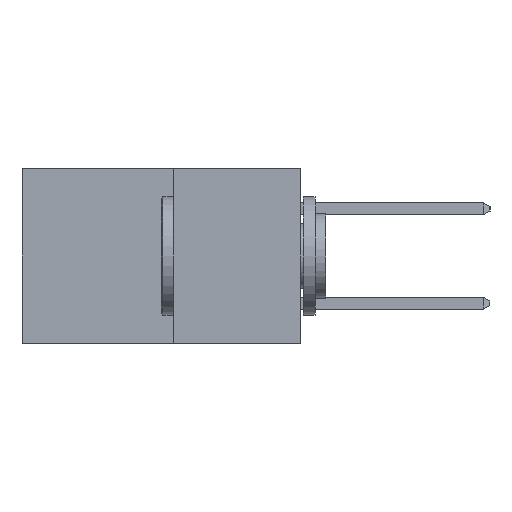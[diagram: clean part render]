
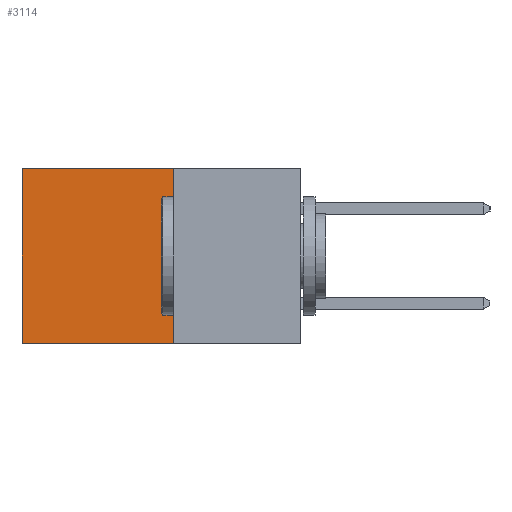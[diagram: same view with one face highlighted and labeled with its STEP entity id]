
A CAD part, left-side view. The second image highlights one B-rep face of the part: STEP entity #3114.
In plain terms, the highlighted planar face has unit normal (-1, 0, 0).
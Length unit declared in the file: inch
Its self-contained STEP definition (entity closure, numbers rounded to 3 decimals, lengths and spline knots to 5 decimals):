
#62 = VECTOR ( 'NONE', #9795, 39.37008 ) ;
#97 = CARTESIAN_POINT ( 'NONE',  ( 0.277, 0.27, -0.37 ) ) ;
#156 = DIRECTION ( 'NONE',  ( 0., 0., -1. ) ) ;
#179 = VECTOR ( 'NONE', #2696, 39.37008 ) ;
#274 = AXIS2_PLACEMENT_3D ( 'NONE', #14590, #12447, #7256 ) ;
#507 = CARTESIAN_POINT ( 'NONE',  ( 0.277, 0.27, -0.37 ) ) ;
#1178 = CARTESIAN_POINT ( 'NONE',  ( 0.277, 0.59, 0. ) ) ;
#2025 = CARTESIAN_POINT ( 'NONE',  ( 0.277, 0.59, -0.37 ) ) ;
#2440 = CARTESIAN_POINT ( 'NONE',  ( 0.277, 0.59, -0.37 ) ) ;
#2696 = DIRECTION ( 'NONE',  ( 0., 1., 0. ) ) ;
#2779 = DIRECTION ( 'NONE',  ( 0., 0., -1. ) ) ;
#2876 = LINE ( 'NONE', #10697, #179 ) ;
#2904 = ORIENTED_EDGE ( 'NONE', *, *, #7811, .T. ) ;
#3114 = ADVANCED_FACE ( 'NONE', ( #4522 ), #6682, .F. ) ;
#3620 = VERTEX_POINT ( 'NONE', #12195 ) ;
#3738 = ORIENTED_EDGE ( 'NONE', *, *, #7316, .F. ) ;
#3823 = EDGE_CURVE ( 'NONE', #11148, #11612, #11852, .T. ) ;
#4067 = ORIENTED_EDGE ( 'NONE', *, *, #11324, .T. ) ;
#4309 = VERTEX_POINT ( 'NONE', #1178 ) ;
#4522 = FACE_OUTER_BOUND ( 'NONE', #14436, .T. ) ;
#5270 = ORIENTED_EDGE ( 'NONE', *, *, #3823, .F. ) ;
#6682 = PLANE ( 'NONE',  #274 ) ;
#7256 = DIRECTION ( 'NONE',  ( 0., 0., -1. ) ) ;
#7316 = EDGE_CURVE ( 'NONE', #3620, #11148, #7692, .T. ) ;
#7692 = LINE ( 'NONE', #507, #13688 ) ;
#7811 = EDGE_CURVE ( 'NONE', #4309, #11612, #10705, .T. ) ;
#9795 = DIRECTION ( 'NONE',  ( 0., 1., 0. ) ) ;
#9821 = CARTESIAN_POINT ( 'NONE',  ( 0.277, 0.27, -0.37 ) ) ;
#10350 = VECTOR ( 'NONE', #156, 39.37008 ) ;
#10697 = CARTESIAN_POINT ( 'NONE',  ( 0.277, 0.27, 0. ) ) ;
#10705 = LINE ( 'NONE', #2440, #10350 ) ;
#11148 = VERTEX_POINT ( 'NONE', #97 ) ;
#11324 = EDGE_CURVE ( 'NONE', #3620, #4309, #2876, .T. ) ;
#11612 = VERTEX_POINT ( 'NONE', #2025 ) ;
#11852 = LINE ( 'NONE', #9821, #62 ) ;
#12195 = CARTESIAN_POINT ( 'NONE',  ( 0.277, 0.27, 0. ) ) ;
#12447 = DIRECTION ( 'NONE',  ( 1., 0., 0. ) ) ;
#13688 = VECTOR ( 'NONE', #2779, 39.37008 ) ;
#14436 = EDGE_LOOP ( 'NONE', ( #2904, #5270, #3738, #4067 ) ) ;
#14590 = CARTESIAN_POINT ( 'NONE',  ( 0.277, 0.27, -0.37 ) ) ;
